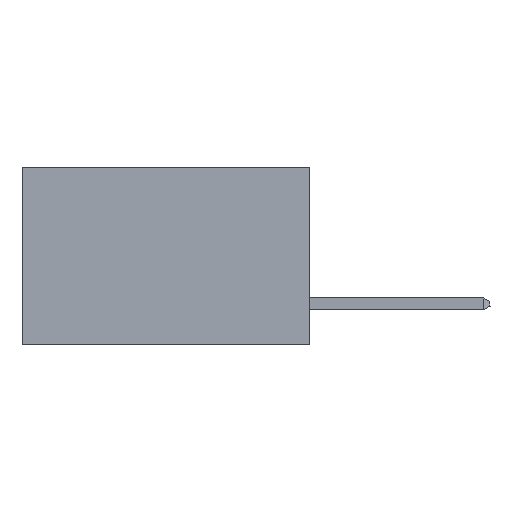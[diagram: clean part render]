
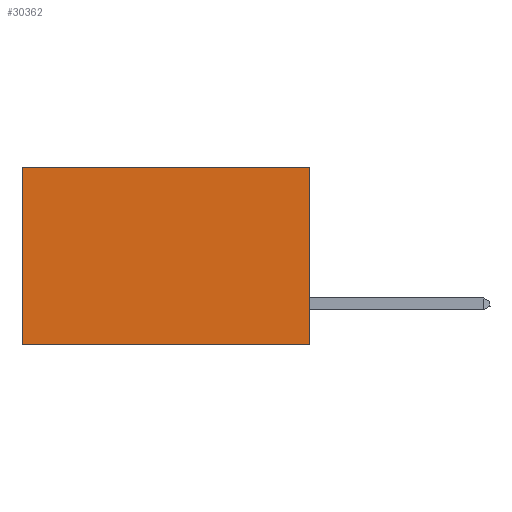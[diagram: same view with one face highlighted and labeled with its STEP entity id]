
A CAD part, left-side view. The second image highlights one B-rep face of the part: STEP entity #30362.
In plain terms, the highlighted planar face has unit normal (-1, 0, 0).
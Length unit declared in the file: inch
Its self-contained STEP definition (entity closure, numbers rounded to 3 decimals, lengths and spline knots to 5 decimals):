
#11 = AXIS2_PLACEMENT_3D ( 'NONE', #14200, #3832, #3481 ) ;
#189 = EDGE_CURVE ( 'NONE', #12609, #31582, #18071, .T. ) ;
#211 = LINE ( 'NONE', #21825, #8747 ) ;
#1742 = VECTOR ( 'NONE', #4407, 39.37008 ) ;
#3481 = DIRECTION ( 'NONE',  ( 0., 0., -1. ) ) ;
#3832 = DIRECTION ( 'NONE',  ( 1., 0., 0. ) ) ;
#4407 = DIRECTION ( 'NONE',  ( 0., 0., -1. ) ) ;
#5848 = CARTESIAN_POINT ( 'NONE',  ( 0.2875, 0., -0.37 ) ) ;
#6183 = PLANE ( 'NONE',  #11 ) ;
#7360 = CARTESIAN_POINT ( 'NONE',  ( 0.2875, 0., 0. ) ) ;
#7372 = DIRECTION ( 'NONE',  ( 0., 1., 0. ) ) ;
#7380 = ORIENTED_EDGE ( 'NONE', *, *, #23211, .F. ) ;
#8747 = VECTOR ( 'NONE', #24810, 39.37008 ) ;
#9027 = LINE ( 'NONE', #22594, #1742 ) ;
#9204 = CARTESIAN_POINT ( 'NONE',  ( 0.2875, 0.6, -0.37 ) ) ;
#12212 = EDGE_LOOP ( 'NONE', ( #30504, #25178, #7380, #29260 ) ) ;
#12448 = EDGE_CURVE ( 'NONE', #20403, #19205, #22159, .T. ) ;
#12609 = VERTEX_POINT ( 'NONE', #5848 ) ;
#14200 = CARTESIAN_POINT ( 'NONE',  ( 0.2875, 0., 0. ) ) ;
#14779 = VECTOR ( 'NONE', #7372, 39.37008 ) ;
#18071 = LINE ( 'NONE', #33014, #14779 ) ;
#19205 = VERTEX_POINT ( 'NONE', #24767 ) ;
#19218 = VECTOR ( 'NONE', #21551, 39.37008 ) ;
#20403 = VERTEX_POINT ( 'NONE', #21624 ) ;
#21551 = DIRECTION ( 'NONE',  ( 0., 1., 0. ) ) ;
#21624 = CARTESIAN_POINT ( 'NONE',  ( 0.2875, 0., 0. ) ) ;
#21825 = CARTESIAN_POINT ( 'NONE',  ( 0.2875, 0., 0. ) ) ;
#22159 = LINE ( 'NONE', #7360, #19218 ) ;
#22594 = CARTESIAN_POINT ( 'NONE',  ( 0.2875, 0.6, 0. ) ) ;
#23211 = EDGE_CURVE ( 'NONE', #20403, #12609, #211, .T. ) ;
#24767 = CARTESIAN_POINT ( 'NONE',  ( 0.2875, 0.6, 0. ) ) ;
#24810 = DIRECTION ( 'NONE',  ( 0., 0., -1. ) ) ;
#25178 = ORIENTED_EDGE ( 'NONE', *, *, #189, .F. ) ;
#25558 = EDGE_CURVE ( 'NONE', #19205, #31582, #9027, .T. ) ;
#29260 = ORIENTED_EDGE ( 'NONE', *, *, #12448, .T. ) ;
#30362 = ADVANCED_FACE ( 'NONE', ( #31552 ), #6183, .F. ) ;
#30504 = ORIENTED_EDGE ( 'NONE', *, *, #25558, .T. ) ;
#31552 = FACE_OUTER_BOUND ( 'NONE', #12212, .T. ) ;
#31582 = VERTEX_POINT ( 'NONE', #9204 ) ;
#33014 = CARTESIAN_POINT ( 'NONE',  ( 0.2875, 0., -0.37 ) ) ;
